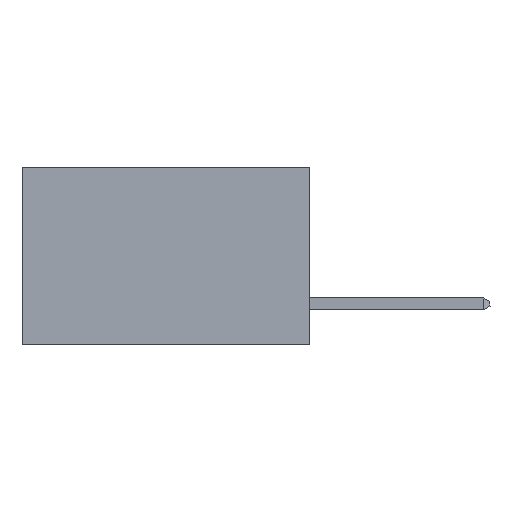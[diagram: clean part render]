
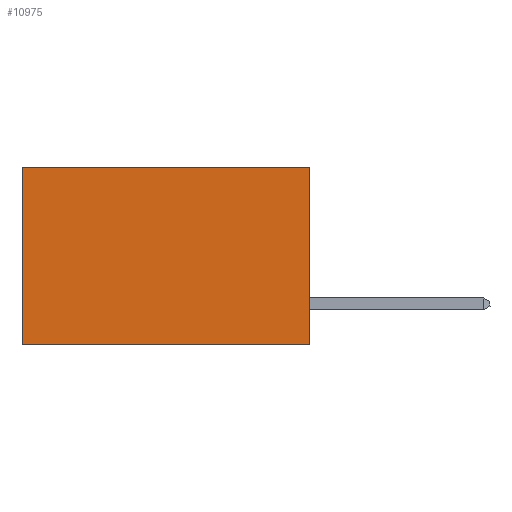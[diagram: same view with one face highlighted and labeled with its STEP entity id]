
A CAD part, left-side view. The second image highlights one B-rep face of the part: STEP entity #10975.
In plain terms, the highlighted planar face has unit normal (-1, 0, 0).
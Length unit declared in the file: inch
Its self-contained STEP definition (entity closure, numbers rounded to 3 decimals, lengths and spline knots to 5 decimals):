
#615 = CARTESIAN_POINT ( 'NONE',  ( 0.2875, 0., 0. ) ) ;
#667 = EDGE_LOOP ( 'NONE', ( #2472, #4438, #9097, #2111 ) ) ;
#976 = CARTESIAN_POINT ( 'NONE',  ( 0.2875, 0.6, 0. ) ) ;
#1076 = CARTESIAN_POINT ( 'NONE',  ( 0.2875, 0.6, -0.37 ) ) ;
#1627 = VERTEX_POINT ( 'NONE', #976 ) ;
#2111 = ORIENTED_EDGE ( 'NONE', *, *, #7080, .T. ) ;
#2472 = ORIENTED_EDGE ( 'NONE', *, *, #4053, .T. ) ;
#2703 = CARTESIAN_POINT ( 'NONE',  ( 0.2875, 0., 0. ) ) ;
#2711 = LINE ( 'NONE', #9679, #10283 ) ;
#2871 = DIRECTION ( 'NONE',  ( 0., 0., -1. ) ) ;
#3444 = DIRECTION ( 'NONE',  ( 0., 1., 0. ) ) ;
#3733 = EDGE_CURVE ( 'NONE', #9801, #11299, #8697, .T. ) ;
#3847 = PLANE ( 'NONE',  #8301 ) ;
#4053 = EDGE_CURVE ( 'NONE', #1627, #8141, #4333, .T. ) ;
#4225 = CARTESIAN_POINT ( 'NONE',  ( 0.2875, 0., -0.37 ) ) ;
#4333 = LINE ( 'NONE', #4585, #8831 ) ;
#4438 = ORIENTED_EDGE ( 'NONE', *, *, #8159, .F. ) ;
#4585 = CARTESIAN_POINT ( 'NONE',  ( 0.2875, 0.6, 0. ) ) ;
#5606 = CARTESIAN_POINT ( 'NONE',  ( 0.2875, 0., 0. ) ) ;
#5833 = FACE_OUTER_BOUND ( 'NONE', #667, .T. ) ;
#6170 = VECTOR ( 'NONE', #10841, 39.37008 ) ;
#6284 = DIRECTION ( 'NONE',  ( 0., 0., -1. ) ) ;
#6439 = CARTESIAN_POINT ( 'NONE',  ( 0.2875, 0., -0.37 ) ) ;
#7080 = EDGE_CURVE ( 'NONE', #9801, #1627, #2711, .T. ) ;
#7812 = LINE ( 'NONE', #6439, #6170 ) ;
#8141 = VERTEX_POINT ( 'NONE', #1076 ) ;
#8159 = EDGE_CURVE ( 'NONE', #11299, #8141, #7812, .T. ) ;
#8301 = AXIS2_PLACEMENT_3D ( 'NONE', #5606, #9249, #2871 ) ;
#8697 = LINE ( 'NONE', #615, #9841 ) ;
#8831 = VECTOR ( 'NONE', #6284, 39.37008 ) ;
#9097 = ORIENTED_EDGE ( 'NONE', *, *, #3733, .F. ) ;
#9249 = DIRECTION ( 'NONE',  ( 1., 0., 0. ) ) ;
#9561 = DIRECTION ( 'NONE',  ( 0., 0., -1. ) ) ;
#9679 = CARTESIAN_POINT ( 'NONE',  ( 0.2875, 0., 0. ) ) ;
#9801 = VERTEX_POINT ( 'NONE', #2703 ) ;
#9841 = VECTOR ( 'NONE', #9561, 39.37008 ) ;
#10283 = VECTOR ( 'NONE', #3444, 39.37008 ) ;
#10841 = DIRECTION ( 'NONE',  ( 0., 1., 0. ) ) ;
#10975 = ADVANCED_FACE ( 'NONE', ( #5833 ), #3847, .F. ) ;
#11299 = VERTEX_POINT ( 'NONE', #4225 ) ;
